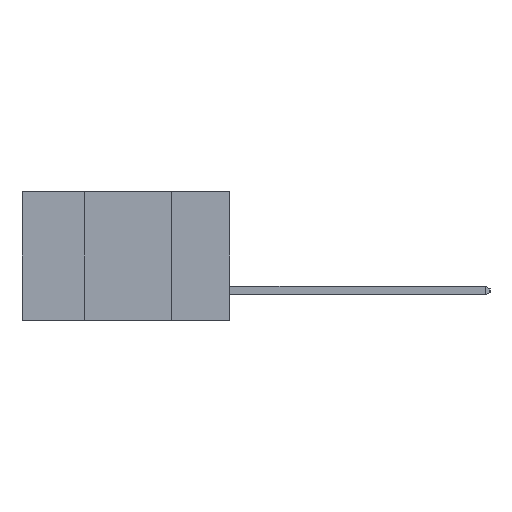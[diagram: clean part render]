
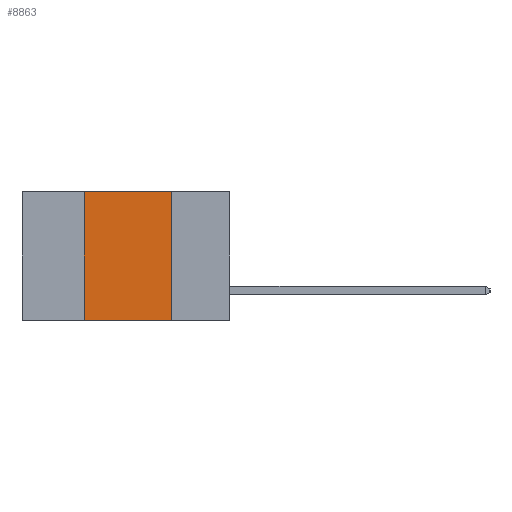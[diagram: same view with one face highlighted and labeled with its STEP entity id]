
A CAD part, left-side view. The second image highlights one B-rep face of the part: STEP entity #8863.
In plain terms, the highlighted planar face has unit normal (-1, 0, 0).
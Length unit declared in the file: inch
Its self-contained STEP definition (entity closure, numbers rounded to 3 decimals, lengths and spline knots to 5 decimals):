
#554 = FACE_OUTER_BOUND ( 'NONE', #7913, .T. ) ;
#1013 = DIRECTION ( 'NONE',  ( 0., 0., -1. ) ) ;
#1093 = EDGE_CURVE ( 'NONE', #5036, #11444, #5181, .T. ) ;
#1182 = VERTEX_POINT ( 'NONE', #2668 ) ;
#1333 = CARTESIAN_POINT ( 'NONE',  ( 0., 0.6, 0. ) ) ;
#1502 = CARTESIAN_POINT ( 'NONE',  ( 0., 0.17, -0.37 ) ) ;
#1559 = DIRECTION ( 'NONE',  ( 0., -1., 0. ) ) ;
#1862 = EDGE_CURVE ( 'NONE', #1182, #11350, #3926, .T. ) ;
#2668 = CARTESIAN_POINT ( 'NONE',  ( 0., 0.17, 0. ) ) ;
#2708 = CARTESIAN_POINT ( 'NONE',  ( 0., 0.17, -0.37 ) ) ;
#2763 = PLANE ( 'NONE',  #3889 ) ;
#2821 = VECTOR ( 'NONE', #5780, 39.37008 ) ;
#3217 = ORIENTED_EDGE ( 'NONE', *, *, #5164, .T. ) ;
#3234 = VECTOR ( 'NONE', #1559, 39.37008 ) ;
#3808 = DIRECTION ( 'NONE',  ( 0., -1., 0. ) ) ;
#3850 = CARTESIAN_POINT ( 'NONE',  ( 0., 0.6, -0.37 ) ) ;
#3889 = AXIS2_PLACEMENT_3D ( 'NONE', #4796, #11933, #5783 ) ;
#3898 = EDGE_CURVE ( 'NONE', #11444, #1182, #8681, .T. ) ;
#3926 = LINE ( 'NONE', #1502, #9069 ) ;
#4618 = VECTOR ( 'NONE', #3808, 39.37008 ) ;
#4796 = CARTESIAN_POINT ( 'NONE',  ( 0., 0.6, 0. ) ) ;
#4951 = LINE ( 'NONE', #3850, #4618 ) ;
#5036 = VERTEX_POINT ( 'NONE', #6159 ) ;
#5164 = EDGE_CURVE ( 'NONE', #5036, #11350, #4951, .T. ) ;
#5181 = LINE ( 'NONE', #5884, #2821 ) ;
#5247 = ORIENTED_EDGE ( 'NONE', *, *, #1093, .F. ) ;
#5780 = DIRECTION ( 'NONE',  ( 0., 0., 1. ) ) ;
#5783 = DIRECTION ( 'NONE',  ( 0., 0., -1. ) ) ;
#5884 = CARTESIAN_POINT ( 'NONE',  ( 0., 0.42, -0.37 ) ) ;
#6159 = CARTESIAN_POINT ( 'NONE',  ( 0., 0.42, -0.37 ) ) ;
#6905 = ORIENTED_EDGE ( 'NONE', *, *, #3898, .F. ) ;
#7913 = EDGE_LOOP ( 'NONE', ( #12729, #6905, #5247, #3217 ) ) ;
#8681 = LINE ( 'NONE', #1333, #3234 ) ;
#8863 = ADVANCED_FACE ( 'NONE', ( #554 ), #2763, .F. ) ;
#9069 = VECTOR ( 'NONE', #1013, 39.37008 ) ;
#11350 = VERTEX_POINT ( 'NONE', #2708 ) ;
#11444 = VERTEX_POINT ( 'NONE', #12960 ) ;
#11933 = DIRECTION ( 'NONE',  ( 1., 0., 0. ) ) ;
#12729 = ORIENTED_EDGE ( 'NONE', *, *, #1862, .F. ) ;
#12960 = CARTESIAN_POINT ( 'NONE',  ( 0., 0.42, 0. ) ) ;
